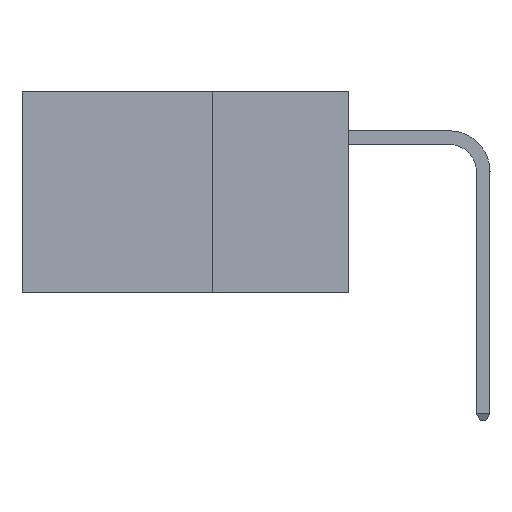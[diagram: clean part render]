
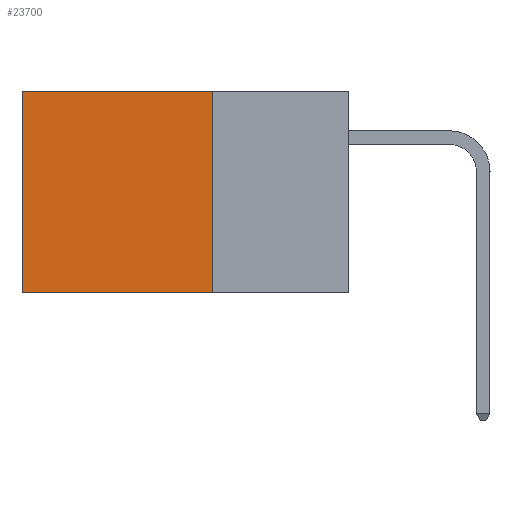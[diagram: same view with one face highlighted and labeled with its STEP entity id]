
A CAD part, left-side view. The second image highlights one B-rep face of the part: STEP entity #23700.
In plain terms, the highlighted planar face has unit normal (-1, 0, 0).
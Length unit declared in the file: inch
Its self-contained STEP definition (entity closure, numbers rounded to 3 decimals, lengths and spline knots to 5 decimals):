
#581 = VERTEX_POINT ( 'NONE', #13654 ) ;
#862 = ORIENTED_EDGE ( 'NONE', *, *, #2149, .F. ) ;
#2039 = EDGE_CURVE ( 'NONE', #19745, #26557, #6558, .T. ) ;
#2149 = EDGE_CURVE ( 'NONE', #26557, #12835, #34758, .T. ) ;
#3536 = CARTESIAN_POINT ( 'NONE',  ( 0.2875, 0.6, -0.37 ) ) ;
#6092 = CARTESIAN_POINT ( 'NONE',  ( 0.2875, 0.25, -0.37 ) ) ;
#6558 = LINE ( 'NONE', #31136, #37500 ) ;
#11318 = ORIENTED_EDGE ( 'NONE', *, *, #24415, .T. ) ;
#11678 = PLANE ( 'NONE',  #37299 ) ;
#12472 = VECTOR ( 'NONE', #17994, 39.37008 ) ;
#12826 = CARTESIAN_POINT ( 'NONE',  ( 0.2875, 0.25, 0. ) ) ;
#12835 = VERTEX_POINT ( 'NONE', #3536 ) ;
#13405 = FACE_OUTER_BOUND ( 'NONE', #22405, .T. ) ;
#13435 = LINE ( 'NONE', #14977, #12472 ) ;
#13654 = CARTESIAN_POINT ( 'NONE',  ( 0.2875, 0.6, 0. ) ) ;
#14764 = CARTESIAN_POINT ( 'NONE',  ( 0.2875, 0.25, 0. ) ) ;
#14977 = CARTESIAN_POINT ( 'NONE',  ( 0.2875, 0.25, 0. ) ) ;
#17770 = DIRECTION ( 'NONE',  ( 1., 0., 0. ) ) ;
#17994 = DIRECTION ( 'NONE',  ( 0., 1., 0. ) ) ;
#19745 = VERTEX_POINT ( 'NONE', #12826 ) ;
#19893 = VECTOR ( 'NONE', #37006, 39.37008 ) ;
#22055 = LINE ( 'NONE', #22799, #36890 ) ;
#22405 = EDGE_LOOP ( 'NONE', ( #29005, #862, #29013, #11318 ) ) ;
#22799 = CARTESIAN_POINT ( 'NONE',  ( 0.2875, 0.6, 0. ) ) ;
#23700 = ADVANCED_FACE ( 'NONE', ( #13405 ), #11678, .F. ) ;
#24415 = EDGE_CURVE ( 'NONE', #19745, #581, #13435, .T. ) ;
#25791 = DIRECTION ( 'NONE',  ( 0., 0., -1. ) ) ;
#26557 = VERTEX_POINT ( 'NONE', #6092 ) ;
#28305 = EDGE_CURVE ( 'NONE', #581, #12835, #22055, .T. ) ;
#29005 = ORIENTED_EDGE ( 'NONE', *, *, #28305, .T. ) ;
#29013 = ORIENTED_EDGE ( 'NONE', *, *, #2039, .F. ) ;
#31136 = CARTESIAN_POINT ( 'NONE',  ( 0.2875, 0.25, 0. ) ) ;
#34448 = DIRECTION ( 'NONE',  ( 0., 0., -1. ) ) ;
#34758 = LINE ( 'NONE', #37251, #19893 ) ;
#36890 = VECTOR ( 'NONE', #25791, 39.37008 ) ;
#37006 = DIRECTION ( 'NONE',  ( 0., 1., 0. ) ) ;
#37251 = CARTESIAN_POINT ( 'NONE',  ( 0.2875, 0.25, -0.37 ) ) ;
#37299 = AXIS2_PLACEMENT_3D ( 'NONE', #14764, #17770, #38493 ) ;
#37500 = VECTOR ( 'NONE', #34448, 39.37008 ) ;
#38493 = DIRECTION ( 'NONE',  ( 0., 0., -1. ) ) ;
